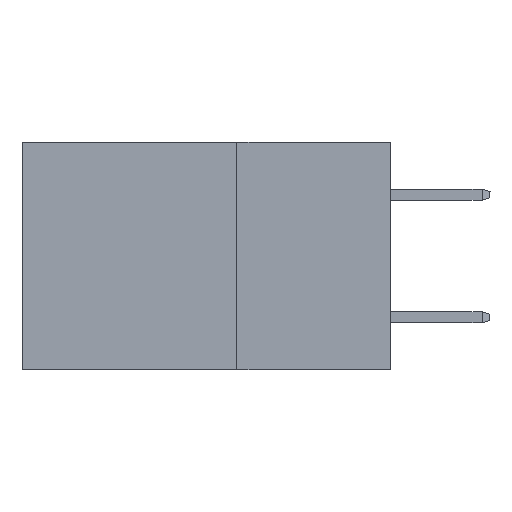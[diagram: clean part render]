
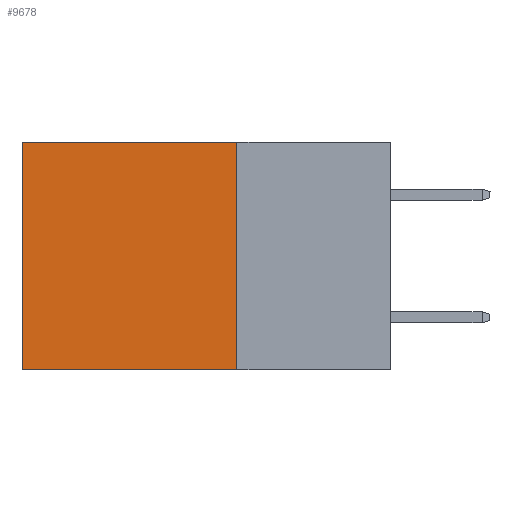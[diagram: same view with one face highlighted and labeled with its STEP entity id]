
A CAD part, left-side view. The second image highlights one B-rep face of the part: STEP entity #9678.
In plain terms, the highlighted planar face has unit normal (-1, 0, 0).
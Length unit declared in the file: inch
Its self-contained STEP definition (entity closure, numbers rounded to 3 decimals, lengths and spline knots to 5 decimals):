
#589 = VERTEX_POINT ( 'NONE', #7004 ) ;
#1128 = VECTOR ( 'NONE', #41297, 39.37008 ) ;
#1967 = CARTESIAN_POINT ( 'NONE',  ( 0.2875, 0.25, 0. ) ) ;
#2912 = VERTEX_POINT ( 'NONE', #15515 ) ;
#3811 = EDGE_CURVE ( 'NONE', #589, #5778, #37367, .T. ) ;
#5778 = VERTEX_POINT ( 'NONE', #25684 ) ;
#6181 = ORIENTED_EDGE ( 'NONE', *, *, #41481, .F. ) ;
#7004 = CARTESIAN_POINT ( 'NONE',  ( 0.2875, 0.25, -0.37 ) ) ;
#7916 = CARTESIAN_POINT ( 'NONE',  ( 0.2875, 0.25, 0. ) ) ;
#7970 = DIRECTION ( 'NONE',  ( 0., 0., -1. ) ) ;
#8358 = EDGE_CURVE ( 'NONE', #2912, #37433, #10524, .T. ) ;
#9330 = VECTOR ( 'NONE', #33224, 39.37008 ) ;
#9678 = ADVANCED_FACE ( 'NONE', ( #13721 ), #17069, .F. ) ;
#10524 = LINE ( 'NONE', #1967, #1128 ) ;
#11611 = CARTESIAN_POINT ( 'NONE',  ( 0.2875, 0.6, 0. ) ) ;
#13389 = VECTOR ( 'NONE', #25535, 39.37008 ) ;
#13721 = FACE_OUTER_BOUND ( 'NONE', #38972, .T. ) ;
#14922 = CARTESIAN_POINT ( 'NONE',  ( 0.2875, 0.25, -0.37 ) ) ;
#15515 = CARTESIAN_POINT ( 'NONE',  ( 0.2875, 0.25, 0. ) ) ;
#16229 = CARTESIAN_POINT ( 'NONE',  ( 0.2875, 0.6, 0. ) ) ;
#16326 = LINE ( 'NONE', #16229, #24529 ) ;
#17069 = PLANE ( 'NONE',  #41888 ) ;
#22486 = DIRECTION ( 'NONE',  ( 1., 0., 0. ) ) ;
#24529 = VECTOR ( 'NONE', #44176, 39.37008 ) ;
#25508 = ORIENTED_EDGE ( 'NONE', *, *, #3811, .F. ) ;
#25535 = DIRECTION ( 'NONE',  ( 0., 0., -1. ) ) ;
#25684 = CARTESIAN_POINT ( 'NONE',  ( 0.2875, 0.6, -0.37 ) ) ;
#29498 = ORIENTED_EDGE ( 'NONE', *, *, #8358, .T. ) ;
#29806 = EDGE_CURVE ( 'NONE', #37433, #5778, #16326, .T. ) ;
#33224 = DIRECTION ( 'NONE',  ( 0., 1., 0. ) ) ;
#37367 = LINE ( 'NONE', #14922, #9330 ) ;
#37433 = VERTEX_POINT ( 'NONE', #11611 ) ;
#38972 = EDGE_LOOP ( 'NONE', ( #42894, #25508, #6181, #29498 ) ) ;
#39492 = CARTESIAN_POINT ( 'NONE',  ( 0.2875, 0.25, 0. ) ) ;
#41297 = DIRECTION ( 'NONE',  ( 0., 1., 0. ) ) ;
#41309 = LINE ( 'NONE', #7916, #13389 ) ;
#41481 = EDGE_CURVE ( 'NONE', #2912, #589, #41309, .T. ) ;
#41888 = AXIS2_PLACEMENT_3D ( 'NONE', #39492, #22486, #7970 ) ;
#42894 = ORIENTED_EDGE ( 'NONE', *, *, #29806, .T. ) ;
#44176 = DIRECTION ( 'NONE',  ( 0., 0., -1. ) ) ;
